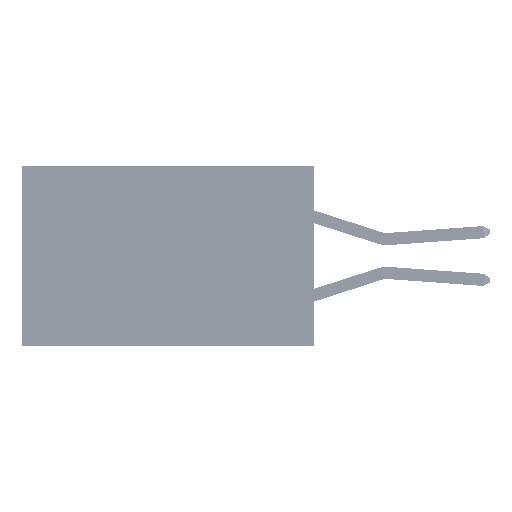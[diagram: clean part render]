
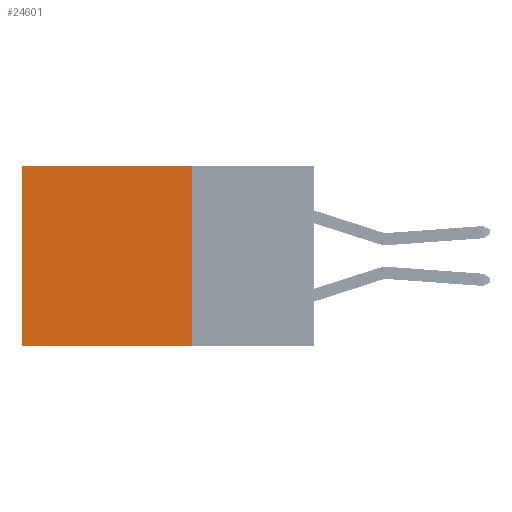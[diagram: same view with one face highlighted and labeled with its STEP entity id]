
A CAD part, left-side view. The second image highlights one B-rep face of the part: STEP entity #24601.
In plain terms, the highlighted planar face has unit normal (-1, 0, 0).
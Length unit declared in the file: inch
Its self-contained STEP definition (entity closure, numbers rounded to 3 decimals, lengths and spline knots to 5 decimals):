
#1104 = ORIENTED_EDGE ( 'NONE', *, *, #1990, .F. ) ;
#1761 = VECTOR ( 'NONE', #48543, 39.37008 ) ;
#1990 = EDGE_CURVE ( 'NONE', #13985, #18148, #35018, .T. ) ;
#2515 = CARTESIAN_POINT ( 'NONE',  ( 0.2875, 0.25, 0. ) ) ;
#3590 = ORIENTED_EDGE ( 'NONE', *, *, #17303, .T. ) ;
#5294 = VERTEX_POINT ( 'NONE', #21510 ) ;
#5473 = DIRECTION ( 'NONE',  ( 1., 0., 0. ) ) ;
#6679 = FACE_OUTER_BOUND ( 'NONE', #28768, .T. ) ;
#8410 = CARTESIAN_POINT ( 'NONE',  ( 0.2875, 0.25, 0. ) ) ;
#12495 = LINE ( 'NONE', #37227, #1761 ) ;
#13985 = VERTEX_POINT ( 'NONE', #2515 ) ;
#14959 = LINE ( 'NONE', #32530, #49314 ) ;
#16300 = DIRECTION ( 'NONE',  ( 0., 0., -1. ) ) ;
#17303 = EDGE_CURVE ( 'NONE', #13985, #40175, #14959, .T. ) ;
#18148 = VERTEX_POINT ( 'NONE', #21703 ) ;
#20226 = AXIS2_PLACEMENT_3D ( 'NONE', #39839, #5473, #28048 ) ;
#21510 = CARTESIAN_POINT ( 'NONE',  ( 0.2875, 0.6, -0.37 ) ) ;
#21703 = CARTESIAN_POINT ( 'NONE',  ( 0.2875, 0.25, -0.37 ) ) ;
#24321 = CARTESIAN_POINT ( 'NONE',  ( 0.2875, 0.6, 0. ) ) ;
#24586 = DIRECTION ( 'NONE',  ( 0., 1., 0. ) ) ;
#24601 = ADVANCED_FACE ( 'NONE', ( #6679 ), #32174, .F. ) ;
#28048 = DIRECTION ( 'NONE',  ( 0., 0., -1. ) ) ;
#28322 = LINE ( 'NONE', #44830, #33607 ) ;
#28768 = EDGE_LOOP ( 'NONE', ( #41502, #31595, #1104, #3590 ) ) ;
#31595 = ORIENTED_EDGE ( 'NONE', *, *, #40864, .F. ) ;
#32174 = PLANE ( 'NONE',  #20226 ) ;
#32530 = CARTESIAN_POINT ( 'NONE',  ( 0.2875, 0.25, 0. ) ) ;
#33607 = VECTOR ( 'NONE', #48001, 39.37008 ) ;
#35018 = LINE ( 'NONE', #8410, #40998 ) ;
#37227 = CARTESIAN_POINT ( 'NONE',  ( 0.2875, 0.6, 0. ) ) ;
#37388 = EDGE_CURVE ( 'NONE', #40175, #5294, #12495, .T. ) ;
#39839 = CARTESIAN_POINT ( 'NONE',  ( 0.2875, 0.25, 0. ) ) ;
#40175 = VERTEX_POINT ( 'NONE', #24321 ) ;
#40864 = EDGE_CURVE ( 'NONE', #18148, #5294, #28322, .T. ) ;
#40998 = VECTOR ( 'NONE', #16300, 39.37008 ) ;
#41502 = ORIENTED_EDGE ( 'NONE', *, *, #37388, .T. ) ;
#44830 = CARTESIAN_POINT ( 'NONE',  ( 0.2875, 0.25, -0.37 ) ) ;
#48001 = DIRECTION ( 'NONE',  ( 0., 1., 0. ) ) ;
#48543 = DIRECTION ( 'NONE',  ( 0., 0., -1. ) ) ;
#49314 = VECTOR ( 'NONE', #24586, 39.37008 ) ;
